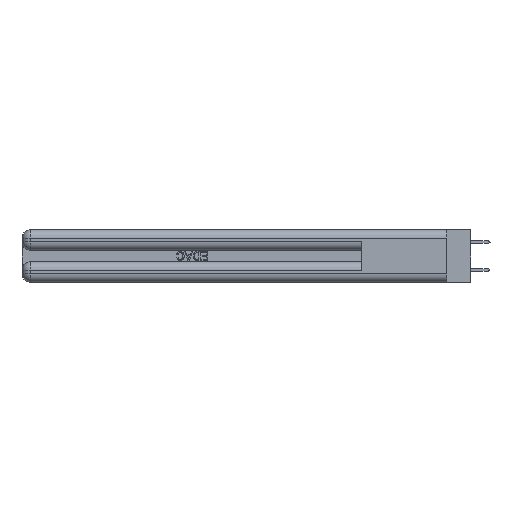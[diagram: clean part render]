
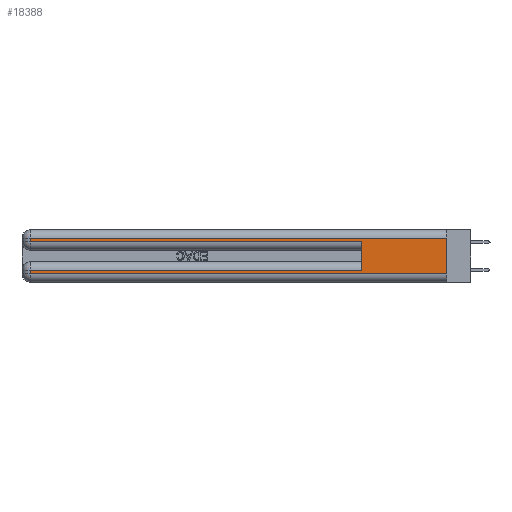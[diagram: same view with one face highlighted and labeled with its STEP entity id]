
A CAD part, left-side view. The second image highlights one B-rep face of the part: STEP entity #18388.
In plain terms, the highlighted planar face has unit normal (-1, 0, 0).
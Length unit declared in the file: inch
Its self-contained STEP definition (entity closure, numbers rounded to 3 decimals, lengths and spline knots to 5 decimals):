
#467 = VECTOR ( 'NONE', #27807, 39.37008 ) ;
#1777 = ORIENTED_EDGE ( 'NONE', *, *, #33517, .T. ) ;
#1866 = EDGE_CURVE ( 'NONE', #45279, #23028, #24174, .T. ) ;
#3752 = EDGE_CURVE ( 'NONE', #19472, #18461, #34478, .T. ) ;
#4014 = CARTESIAN_POINT ( 'NONE',  ( 0., 0., 0.31 ) ) ;
#4836 = AXIS2_PLACEMENT_3D ( 'NONE', #13767, #27830, #41854 ) ;
#4897 = EDGE_CURVE ( 'NONE', #10951, #16645, #38995, .T. ) ;
#5006 = VECTOR ( 'NONE', #39244, 39.37008 ) ;
#5018 = ORIENTED_EDGE ( 'NONE', *, *, #4897, .T. ) ;
#5110 = DIRECTION ( 'NONE',  ( 0., 1., 0. ) ) ;
#5935 = PLANE ( 'NONE',  #4836 ) ;
#7437 = CARTESIAN_POINT ( 'NONE',  ( 0., 2.94, 0.37 ) ) ;
#7758 = CARTESIAN_POINT ( 'NONE',  ( 0., 0.6, 0.285 ) ) ;
#7911 = LINE ( 'NONE', #35782, #27096 ) ;
#8651 = ORIENTED_EDGE ( 'NONE', *, *, #22623, .T. ) ;
#9488 = CARTESIAN_POINT ( 'NONE',  ( 0., 2.94, 0.285 ) ) ;
#10426 = VECTOR ( 'NONE', #26944, 39.37008 ) ;
#10951 = VERTEX_POINT ( 'NONE', #30208 ) ;
#11568 = EDGE_CURVE ( 'NONE', #16645, #18461, #45517, .T. ) ;
#13531 = LINE ( 'NONE', #44160, #42303 ) ;
#13740 = CARTESIAN_POINT ( 'NONE',  ( 0., 0., 0.285 ) ) ;
#13767 = CARTESIAN_POINT ( 'NONE',  ( 0., 0., 0.37 ) ) ;
#16645 = VERTEX_POINT ( 'NONE', #9488 ) ;
#17086 = EDGE_CURVE ( 'NONE', #23028, #18077, #13531, .T. ) ;
#17199 = DIRECTION ( 'NONE',  ( 0., 0., 1. ) ) ;
#18077 = VERTEX_POINT ( 'NONE', #38014 ) ;
#18388 = ADVANCED_FACE ( 'NONE', ( #19761 ), #5935, .F. ) ;
#18461 = VERTEX_POINT ( 'NONE', #7758 ) ;
#19472 = VERTEX_POINT ( 'NONE', #33132 ) ;
#19761 = FACE_OUTER_BOUND ( 'NONE', #29852, .T. ) ;
#20658 = CARTESIAN_POINT ( 'NONE',  ( 0., 0., 0.37 ) ) ;
#21285 = CARTESIAN_POINT ( 'NONE',  ( 0., 0., 0.31 ) ) ;
#22623 = EDGE_CURVE ( 'NONE', #19472, #45279, #7911, .T. ) ;
#23028 = VERTEX_POINT ( 'NONE', #25824 ) ;
#24135 = DIRECTION ( 'NONE',  ( 0., 0., -1. ) ) ;
#24174 = LINE ( 'NONE', #45113, #10426 ) ;
#24774 = ORIENTED_EDGE ( 'NONE', *, *, #11568, .T. ) ;
#25622 = EDGE_CURVE ( 'NONE', #28647, #18077, #28255, .T. ) ;
#25824 = CARTESIAN_POINT ( 'NONE',  ( 0., 2.94, 0.06 ) ) ;
#26944 = DIRECTION ( 'NONE',  ( 0., 0., -1. ) ) ;
#27096 = VECTOR ( 'NONE', #5110, 39.37008 ) ;
#27807 = DIRECTION ( 'NONE',  ( 0., -1., 0. ) ) ;
#27830 = DIRECTION ( 'NONE',  ( 1., 0., 0. ) ) ;
#28255 = LINE ( 'NONE', #20658, #44191 ) ;
#28647 = VERTEX_POINT ( 'NONE', #4014 ) ;
#29852 = EDGE_LOOP ( 'NONE', ( #34179, #1777, #5018, #24774, #38954, #8651, #29991, #36995 ) ) ;
#29991 = ORIENTED_EDGE ( 'NONE', *, *, #1866, .T. ) ;
#30208 = CARTESIAN_POINT ( 'NONE',  ( 0., 2.94, 0.31 ) ) ;
#32611 = VECTOR ( 'NONE', #17199, 39.37008 ) ;
#33132 = CARTESIAN_POINT ( 'NONE',  ( 0., 0.6, 0.085 ) ) ;
#33517 = EDGE_CURVE ( 'NONE', #28647, #10951, #38797, .T. ) ;
#34179 = ORIENTED_EDGE ( 'NONE', *, *, #25622, .F. ) ;
#34478 = LINE ( 'NONE', #34706, #32611 ) ;
#34706 = CARTESIAN_POINT ( 'NONE',  ( 0., 0.6, 0.145 ) ) ;
#35782 = CARTESIAN_POINT ( 'NONE',  ( 0., 0., 0.085 ) ) ;
#36247 = VECTOR ( 'NONE', #41986, 39.37008 ) ;
#36995 = ORIENTED_EDGE ( 'NONE', *, *, #17086, .T. ) ;
#38014 = CARTESIAN_POINT ( 'NONE',  ( 0., 0., 0.06 ) ) ;
#38797 = LINE ( 'NONE', #21285, #5006 ) ;
#38954 = ORIENTED_EDGE ( 'NONE', *, *, #3752, .F. ) ;
#38995 = LINE ( 'NONE', #7437, #36247 ) ;
#39244 = DIRECTION ( 'NONE',  ( 0., 1., 0. ) ) ;
#39291 = CARTESIAN_POINT ( 'NONE',  ( 0., 2.94, 0.085 ) ) ;
#41622 = DIRECTION ( 'NONE',  ( 0., -1., 0. ) ) ;
#41854 = DIRECTION ( 'NONE',  ( 0., 0., -1. ) ) ;
#41986 = DIRECTION ( 'NONE',  ( 0., 0., -1. ) ) ;
#42303 = VECTOR ( 'NONE', #41622, 39.37008 ) ;
#44160 = CARTESIAN_POINT ( 'NONE',  ( 0., 0., 0.06 ) ) ;
#44191 = VECTOR ( 'NONE', #24135, 39.37008 ) ;
#45113 = CARTESIAN_POINT ( 'NONE',  ( 0., 2.94, 0.37 ) ) ;
#45279 = VERTEX_POINT ( 'NONE', #39291 ) ;
#45517 = LINE ( 'NONE', #13740, #467 ) ;
